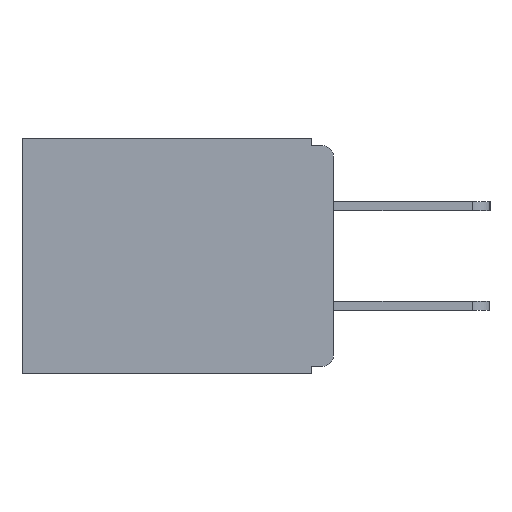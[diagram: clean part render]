
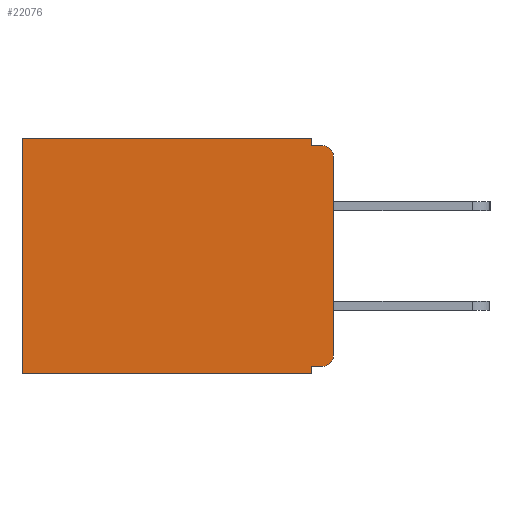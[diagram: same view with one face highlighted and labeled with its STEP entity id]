
A CAD part, left-side view. The second image highlights one B-rep face of the part: STEP entity #22076.
In plain terms, the highlighted planar face has unit normal (-1, 0, 0).
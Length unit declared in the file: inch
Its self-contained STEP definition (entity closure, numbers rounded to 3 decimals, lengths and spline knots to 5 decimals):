
#18 = FACE_OUTER_BOUND ( 'NONE', #20455, .T. ) ;
#424 = ORIENTED_EDGE ( 'NONE', *, *, #19978, .F. ) ;
#998 = CARTESIAN_POINT ( 'NONE',  ( 0.3, 0., -0.01 ) ) ;
#1462 = VERTEX_POINT ( 'NONE', #6685 ) ;
#1550 = LINE ( 'NONE', #13436, #15764 ) ;
#1661 = CARTESIAN_POINT ( 'NONE',  ( 0.3, 0., -0.33 ) ) ;
#1982 = LINE ( 'NONE', #17235, #7793 ) ;
#2110 = VERTEX_POINT ( 'NONE', #16530 ) ;
#2513 = EDGE_CURVE ( 'NONE', #5563, #15599, #16816, .T. ) ;
#2763 = LINE ( 'NONE', #11732, #22472 ) ;
#3267 = DIRECTION ( 'NONE',  ( 0., 0., -1. ) ) ;
#3320 = DIRECTION ( 'NONE',  ( 0., 0., -1. ) ) ;
#3379 = VECTOR ( 'NONE', #12556, 39.37008 ) ;
#3406 = VECTOR ( 'NONE', #3320, 39.37008 ) ;
#3487 = DIRECTION ( 'NONE',  ( -1., 0., 0. ) ) ;
#3626 = CARTESIAN_POINT ( 'NONE',  ( 0.3, 0.015, -0.025 ) ) ;
#3641 = CARTESIAN_POINT ( 'NONE',  ( 0.3, 0.015, -0.305 ) ) ;
#3982 = ORIENTED_EDGE ( 'NONE', *, *, #15191, .F. ) ;
#4597 = AXIS2_PLACEMENT_3D ( 'NONE', #1661, #24508, #9495 ) ;
#5408 = EDGE_CURVE ( 'NONE', #5563, #19565, #23680, .T. ) ;
#5563 = VERTEX_POINT ( 'NONE', #7448 ) ;
#5583 = DIRECTION ( 'NONE',  ( 0., 0., -1. ) ) ;
#5629 = PLANE ( 'NONE',  #4597 ) ;
#5735 = ORIENTED_EDGE ( 'NONE', *, *, #22174, .F. ) ;
#6685 = CARTESIAN_POINT ( 'NONE',  ( 0.3, 0.015, -0.01 ) ) ;
#6808 = CARTESIAN_POINT ( 'NONE',  ( 0.3, 0.437, 0. ) ) ;
#7231 = CARTESIAN_POINT ( 'NONE',  ( 0.3, 0.031, 0. ) ) ;
#7448 = CARTESIAN_POINT ( 'NONE',  ( 0.3, 0.015, -0.32 ) ) ;
#7480 = ORIENTED_EDGE ( 'NONE', *, *, #15339, .T. ) ;
#7608 = DIRECTION ( 'NONE',  ( 0., 1., 0. ) ) ;
#7793 = VECTOR ( 'NONE', #7608, 39.37008 ) ;
#7896 = DIRECTION ( 'NONE',  ( 0., 0., -1. ) ) ;
#8255 = AXIS2_PLACEMENT_3D ( 'NONE', #3641, #3487, #3267 ) ;
#8280 = ORIENTED_EDGE ( 'NONE', *, *, #2513, .F. ) ;
#8467 = DIRECTION ( 'NONE',  ( 0., 0., -1. ) ) ;
#8555 = LINE ( 'NONE', #998, #3379 ) ;
#8582 = LINE ( 'NONE', #7231, #3406 ) ;
#9161 = VERTEX_POINT ( 'NONE', #21210 ) ;
#9495 = DIRECTION ( 'NONE',  ( 0., 0., -1. ) ) ;
#10202 = ORIENTED_EDGE ( 'NONE', *, *, #21221, .T. ) ;
#10237 = CARTESIAN_POINT ( 'NONE',  ( 0.3, 0.437, -0.33 ) ) ;
#10395 = LINE ( 'NONE', #12627, #19956 ) ;
#10605 = AXIS2_PLACEMENT_3D ( 'NONE', #3626, #17070, #5583 ) ;
#11297 = VECTOR ( 'NONE', #8467, 39.37008 ) ;
#11696 = VECTOR ( 'NONE', #18215, 39.37008 ) ;
#11732 = CARTESIAN_POINT ( 'NONE',  ( 0.3, 0., -0.33 ) ) ;
#12556 = DIRECTION ( 'NONE',  ( 0., -1., 0. ) ) ;
#12614 = ORIENTED_EDGE ( 'NONE', *, *, #14588, .F. ) ;
#12627 = CARTESIAN_POINT ( 'NONE',  ( 0.3, 0.437, -0.33 ) ) ;
#13436 = CARTESIAN_POINT ( 'NONE',  ( 0.3, 0., 0. ) ) ;
#14041 = VERTEX_POINT ( 'NONE', #22296 ) ;
#14570 = DIRECTION ( 'NONE',  ( 0., 0., -1. ) ) ;
#14588 = EDGE_CURVE ( 'NONE', #9161, #15043, #1982, .T. ) ;
#14691 = EDGE_CURVE ( 'NONE', #2110, #15474, #8582, .T. ) ;
#14828 = EDGE_CURVE ( 'NONE', #2110, #15180, #1550, .T. ) ;
#15043 = VERTEX_POINT ( 'NONE', #10237 ) ;
#15136 = CIRCLE ( 'NONE', #10605, 0.015 ) ;
#15180 = VERTEX_POINT ( 'NONE', #6808 ) ;
#15191 = EDGE_CURVE ( 'NONE', #15474, #1462, #8555, .T. ) ;
#15339 = EDGE_CURVE ( 'NONE', #14041, #1462, #15136, .T. ) ;
#15474 = VERTEX_POINT ( 'NONE', #21168 ) ;
#15599 = VERTEX_POINT ( 'NONE', #17822 ) ;
#15764 = VECTOR ( 'NONE', #22747, 39.37008 ) ;
#16530 = CARTESIAN_POINT ( 'NONE',  ( 0.3, 0.031, 0. ) ) ;
#16816 = LINE ( 'NONE', #23519, #11696 ) ;
#17070 = DIRECTION ( 'NONE',  ( -1., 0., 0. ) ) ;
#17235 = CARTESIAN_POINT ( 'NONE',  ( 0.3, 0., -0.33 ) ) ;
#17822 = CARTESIAN_POINT ( 'NONE',  ( 0.3, 0.031, -0.32 ) ) ;
#17873 = ORIENTED_EDGE ( 'NONE', *, *, #5408, .T. ) ;
#18011 = CARTESIAN_POINT ( 'NONE',  ( 0.3, 0.031, -0.33 ) ) ;
#18215 = DIRECTION ( 'NONE',  ( 0., 1., 0. ) ) ;
#19565 = VERTEX_POINT ( 'NONE', #22331 ) ;
#19956 = VECTOR ( 'NONE', #14570, 39.37008 ) ;
#19978 = EDGE_CURVE ( 'NONE', #15599, #9161, #24007, .T. ) ;
#20232 = ORIENTED_EDGE ( 'NONE', *, *, #14691, .F. ) ;
#20455 = EDGE_LOOP ( 'NONE', ( #5735, #7480, #3982, #20232, #21736, #10202, #12614, #424, #8280, #17873 ) ) ;
#21168 = CARTESIAN_POINT ( 'NONE',  ( 0.3, 0.031, -0.01 ) ) ;
#21210 = CARTESIAN_POINT ( 'NONE',  ( 0.3, 0.031, -0.33 ) ) ;
#21221 = EDGE_CURVE ( 'NONE', #15180, #15043, #10395, .T. ) ;
#21736 = ORIENTED_EDGE ( 'NONE', *, *, #14828, .T. ) ;
#22076 = ADVANCED_FACE ( 'NONE', ( #18 ), #5629, .F. ) ;
#22174 = EDGE_CURVE ( 'NONE', #14041, #19565, #2763, .T. ) ;
#22296 = CARTESIAN_POINT ( 'NONE',  ( 0.3, 0., -0.025 ) ) ;
#22331 = CARTESIAN_POINT ( 'NONE',  ( 0.3, 0., -0.305 ) ) ;
#22472 = VECTOR ( 'NONE', #7896, 39.37008 ) ;
#22747 = DIRECTION ( 'NONE',  ( 0., 1., 0. ) ) ;
#23519 = CARTESIAN_POINT ( 'NONE',  ( 0.3, 0., -0.32 ) ) ;
#23680 = CIRCLE ( 'NONE', #8255, 0.015 ) ;
#24007 = LINE ( 'NONE', #18011, #11297 ) ;
#24508 = DIRECTION ( 'NONE',  ( 1., 0., 0. ) ) ;
